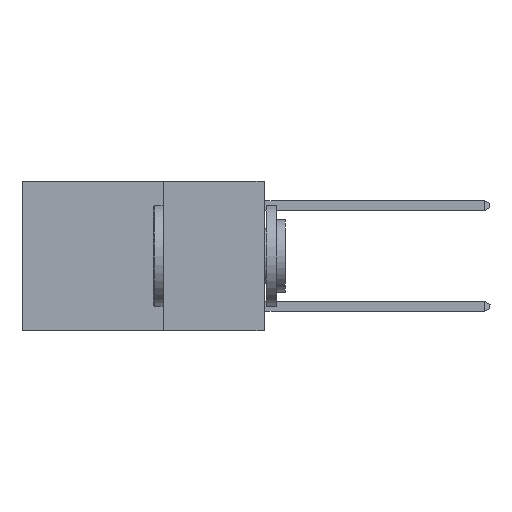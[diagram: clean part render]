
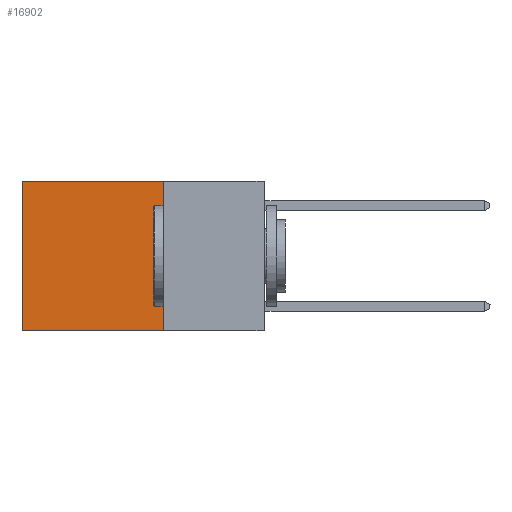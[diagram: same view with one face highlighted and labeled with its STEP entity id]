
A CAD part, left-side view. The second image highlights one B-rep face of the part: STEP entity #16902.
In plain terms, the highlighted planar face has unit normal (-1, 0, 0).
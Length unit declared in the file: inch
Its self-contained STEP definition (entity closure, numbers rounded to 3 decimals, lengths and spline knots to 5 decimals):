
#111 = ORIENTED_EDGE ( 'NONE', *, *, #24425, .F. ) ;
#1088 = CARTESIAN_POINT ( 'NONE',  ( 0.2625, 0.25, 0. ) ) ;
#1273 = CARTESIAN_POINT ( 'NONE',  ( 0.2625, 0.6, 0. ) ) ;
#3640 = FACE_OUTER_BOUND ( 'NONE', #27026, .T. ) ;
#3974 = DIRECTION ( 'NONE',  ( 0., 0., -1. ) ) ;
#4500 = VERTEX_POINT ( 'NONE', #1273 ) ;
#5621 = VECTOR ( 'NONE', #20941, 39.37008 ) ;
#6338 = EDGE_CURVE ( 'NONE', #4500, #18288, #10172, .T. ) ;
#7641 = ORIENTED_EDGE ( 'NONE', *, *, #6338, .T. ) ;
#8201 = EDGE_CURVE ( 'NONE', #17766, #12738, #13983, .T. ) ;
#9601 = EDGE_CURVE ( 'NONE', #17766, #4500, #14154, .T. ) ;
#10172 = LINE ( 'NONE', #20269, #19870 ) ;
#11177 = DIRECTION ( 'NONE',  ( 0., 1., 0. ) ) ;
#12738 = VERTEX_POINT ( 'NONE', #23680 ) ;
#13652 = CARTESIAN_POINT ( 'NONE',  ( 0.2625, 0.25, 0. ) ) ;
#13983 = LINE ( 'NONE', #18949, #5621 ) ;
#14154 = LINE ( 'NONE', #1088, #26835 ) ;
#16902 = ADVANCED_FACE ( 'NONE', ( #3640 ), #18708, .F. ) ;
#17458 = DIRECTION ( 'NONE',  ( 0., 1., 0. ) ) ;
#17766 = VERTEX_POINT ( 'NONE', #13652 ) ;
#18288 = VERTEX_POINT ( 'NONE', #23225 ) ;
#18545 = CARTESIAN_POINT ( 'NONE',  ( 0.2625, 0.25, 0. ) ) ;
#18708 = PLANE ( 'NONE',  #25491 ) ;
#18949 = CARTESIAN_POINT ( 'NONE',  ( 0.2625, 0.25, 0. ) ) ;
#19870 = VECTOR ( 'NONE', #30374, 39.37008 ) ;
#20269 = CARTESIAN_POINT ( 'NONE',  ( 0.2625, 0.6, 0. ) ) ;
#20941 = DIRECTION ( 'NONE',  ( 0., 0., -1. ) ) ;
#20952 = VECTOR ( 'NONE', #17458, 39.37008 ) ;
#21018 = DIRECTION ( 'NONE',  ( 1., 0., 0. ) ) ;
#22745 = CARTESIAN_POINT ( 'NONE',  ( 0.2625, 0.25, -0.37 ) ) ;
#23225 = CARTESIAN_POINT ( 'NONE',  ( 0.2625, 0.6, -0.37 ) ) ;
#23680 = CARTESIAN_POINT ( 'NONE',  ( 0.2625, 0.25, -0.37 ) ) ;
#24425 = EDGE_CURVE ( 'NONE', #12738, #18288, #27396, .T. ) ;
#25267 = ORIENTED_EDGE ( 'NONE', *, *, #9601, .T. ) ;
#25491 = AXIS2_PLACEMENT_3D ( 'NONE', #18545, #21018, #3974 ) ;
#26835 = VECTOR ( 'NONE', #11177, 39.37008 ) ;
#27026 = EDGE_LOOP ( 'NONE', ( #7641, #111, #29946, #25267 ) ) ;
#27396 = LINE ( 'NONE', #22745, #20952 ) ;
#29946 = ORIENTED_EDGE ( 'NONE', *, *, #8201, .F. ) ;
#30374 = DIRECTION ( 'NONE',  ( 0., 0., -1. ) ) ;
